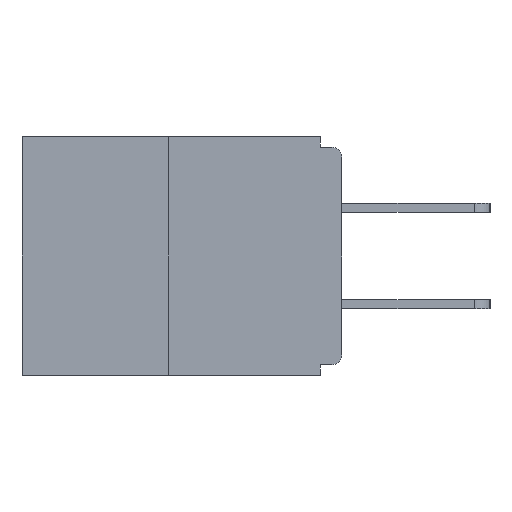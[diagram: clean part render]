
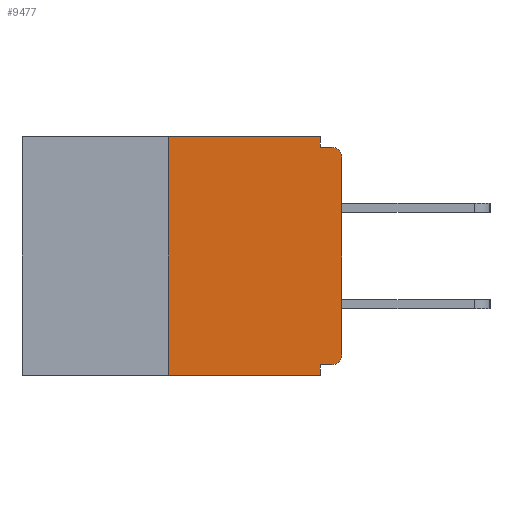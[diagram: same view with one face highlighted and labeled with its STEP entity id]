
A CAD part, left-side view. The second image highlights one B-rep face of the part: STEP entity #9477.
In plain terms, the highlighted planar face has unit normal (-1, 0, 0).
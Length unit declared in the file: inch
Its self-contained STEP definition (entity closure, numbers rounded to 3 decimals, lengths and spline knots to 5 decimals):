
#110 = VERTEX_POINT ( 'NONE', #1755 ) ;
#421 = ORIENTED_EDGE ( 'NONE', *, *, #6780, .F. ) ;
#756 = ORIENTED_EDGE ( 'NONE', *, *, #4641, .T. ) ;
#833 = VECTOR ( 'NONE', #8830, 39.37008 ) ;
#1024 = LINE ( 'NONE', #13984, #12676 ) ;
#1344 = DIRECTION ( 'NONE',  ( 0., -1., 0. ) ) ;
#1395 = DIRECTION ( 'NONE',  ( 0., 0., 1. ) ) ;
#1589 = EDGE_CURVE ( 'NONE', #13357, #110, #1593, .T. ) ;
#1593 = LINE ( 'NONE', #5989, #12550 ) ;
#1641 = VERTEX_POINT ( 'NONE', #7124 ) ;
#1755 = CARTESIAN_POINT ( 'NONE',  ( 0., 0.031, 0. ) ) ;
#1985 = CARTESIAN_POINT ( 'NONE',  ( 0., 0.25, -0.343 ) ) ;
#2175 = LINE ( 'NONE', #6427, #5688 ) ;
#2396 = ORIENTED_EDGE ( 'NONE', *, *, #7268, .T. ) ;
#2651 = EDGE_LOOP ( 'NONE', ( #11910, #13180, #756, #8255, #13586, #6016, #5968, #2396, #421, #5156 ) ) ;
#2699 = DIRECTION ( 'NONE',  ( -1., 0., 0. ) ) ;
#2828 = FACE_OUTER_BOUND ( 'NONE', #2651, .T. ) ;
#3337 = DIRECTION ( 'NONE',  ( 0., 0., -1. ) ) ;
#4010 = CARTESIAN_POINT ( 'NONE',  ( 0., 0.015, -0.313 ) ) ;
#4027 = PLANE ( 'NONE',  #7865 ) ;
#4117 = DIRECTION ( 'NONE',  ( 0., -1., 0. ) ) ;
#4166 = LINE ( 'NONE', #4660, #11087 ) ;
#4237 = CARTESIAN_POINT ( 'NONE',  ( 0., 0.015, -0.328 ) ) ;
#4283 = EDGE_CURVE ( 'NONE', #10764, #13357, #1024, .T. ) ;
#4341 = CARTESIAN_POINT ( 'NONE',  ( 0., 0.031, 0. ) ) ;
#4602 = DIRECTION ( 'NONE',  ( 1., 0., 0. ) ) ;
#4641 = EDGE_CURVE ( 'NONE', #10764, #9894, #5731, .T. ) ;
#4660 = CARTESIAN_POINT ( 'NONE',  ( 0., 0., -0.015 ) ) ;
#4805 = CARTESIAN_POINT ( 'NONE',  ( 0., 0., -0.313 ) ) ;
#4920 = LINE ( 'NONE', #11640, #14516 ) ;
#5156 = ORIENTED_EDGE ( 'NONE', *, *, #8084, .F. ) ;
#5164 = CIRCLE ( 'NONE', #12376, 0.015 ) ;
#5212 = DIRECTION ( 'NONE',  ( 0., 0., -1. ) ) ;
#5361 = LINE ( 'NONE', #4341, #9454 ) ;
#5688 = VECTOR ( 'NONE', #12239, 39.37008 ) ;
#5731 = LINE ( 'NONE', #6086, #13027 ) ;
#5968 = ORIENTED_EDGE ( 'NONE', *, *, #11249, .T. ) ;
#5989 = CARTESIAN_POINT ( 'NONE',  ( 0., 0.46, 0. ) ) ;
#6016 = ORIENTED_EDGE ( 'NONE', *, *, #6105, .T. ) ;
#6086 = CARTESIAN_POINT ( 'NONE',  ( 0., 0.46, -0.343 ) ) ;
#6105 = EDGE_CURVE ( 'NONE', #11072, #11802, #5164, .T. ) ;
#6158 = CARTESIAN_POINT ( 'NONE',  ( 0., 0.031, -0.328 ) ) ;
#6427 = CARTESIAN_POINT ( 'NONE',  ( 0., 0., -0.328 ) ) ;
#6776 = LINE ( 'NONE', #9566, #833 ) ;
#6780 = EDGE_CURVE ( 'NONE', #10482, #1641, #4166, .T. ) ;
#7124 = CARTESIAN_POINT ( 'NONE',  ( 0., 0.015, -0.015 ) ) ;
#7268 = EDGE_CURVE ( 'NONE', #13311, #1641, #9836, .T. ) ;
#7865 = AXIS2_PLACEMENT_3D ( 'NONE', #11270, #4602, #9106 ) ;
#8084 = EDGE_CURVE ( 'NONE', #110, #10482, #5361, .T. ) ;
#8098 = DIRECTION ( 'NONE',  ( 0., -1., 0. ) ) ;
#8255 = ORIENTED_EDGE ( 'NONE', *, *, #13496, .F. ) ;
#8388 = EDGE_CURVE ( 'NONE', #11072, #10570, #2175, .T. ) ;
#8830 = DIRECTION ( 'NONE',  ( 0., 0., -1. ) ) ;
#9106 = DIRECTION ( 'NONE',  ( 0., 0., -1. ) ) ;
#9454 = VECTOR ( 'NONE', #3337, 39.37008 ) ;
#9477 = ADVANCED_FACE ( 'NONE', ( #2828 ), #4027, .F. ) ;
#9566 = CARTESIAN_POINT ( 'NONE',  ( 0., 0.031, -0.343 ) ) ;
#9836 = CIRCLE ( 'NONE', #11515, 0.015 ) ;
#9894 = VERTEX_POINT ( 'NONE', #13308 ) ;
#10164 = CARTESIAN_POINT ( 'NONE',  ( 0., 0., -0.03 ) ) ;
#10482 = VERTEX_POINT ( 'NONE', #12715 ) ;
#10570 = VERTEX_POINT ( 'NONE', #6158 ) ;
#10764 = VERTEX_POINT ( 'NONE', #1985 ) ;
#10929 = DIRECTION ( 'NONE',  ( -1., 0., 0. ) ) ;
#11072 = VERTEX_POINT ( 'NONE', #4237 ) ;
#11087 = VECTOR ( 'NONE', #8098, 39.37008 ) ;
#11249 = EDGE_CURVE ( 'NONE', #11802, #13311, #4920, .T. ) ;
#11270 = CARTESIAN_POINT ( 'NONE',  ( 0., 0.46, 0. ) ) ;
#11515 = AXIS2_PLACEMENT_3D ( 'NONE', #12817, #2699, #14094 ) ;
#11640 = CARTESIAN_POINT ( 'NONE',  ( 0., 0., 0. ) ) ;
#11802 = VERTEX_POINT ( 'NONE', #4805 ) ;
#11910 = ORIENTED_EDGE ( 'NONE', *, *, #1589, .F. ) ;
#12239 = DIRECTION ( 'NONE',  ( 0., 1., 0. ) ) ;
#12376 = AXIS2_PLACEMENT_3D ( 'NONE', #4010, #10929, #5212 ) ;
#12550 = VECTOR ( 'NONE', #1344, 39.37008 ) ;
#12676 = VECTOR ( 'NONE', #1395, 39.37008 ) ;
#12715 = CARTESIAN_POINT ( 'NONE',  ( 0., 0.031, -0.015 ) ) ;
#12777 = DIRECTION ( 'NONE',  ( 0., 0., 1. ) ) ;
#12817 = CARTESIAN_POINT ( 'NONE',  ( 0., 0.015, -0.03 ) ) ;
#13027 = VECTOR ( 'NONE', #4117, 39.37008 ) ;
#13180 = ORIENTED_EDGE ( 'NONE', *, *, #4283, .F. ) ;
#13308 = CARTESIAN_POINT ( 'NONE',  ( 0., 0.031, -0.343 ) ) ;
#13311 = VERTEX_POINT ( 'NONE', #10164 ) ;
#13357 = VERTEX_POINT ( 'NONE', #13665 ) ;
#13496 = EDGE_CURVE ( 'NONE', #10570, #9894, #6776, .T. ) ;
#13586 = ORIENTED_EDGE ( 'NONE', *, *, #8388, .F. ) ;
#13665 = CARTESIAN_POINT ( 'NONE',  ( 0., 0.25, 0. ) ) ;
#13984 = CARTESIAN_POINT ( 'NONE',  ( 0., 0.25, 0. ) ) ;
#14094 = DIRECTION ( 'NONE',  ( 0., 0., -1. ) ) ;
#14516 = VECTOR ( 'NONE', #12777, 39.37008 ) ;
